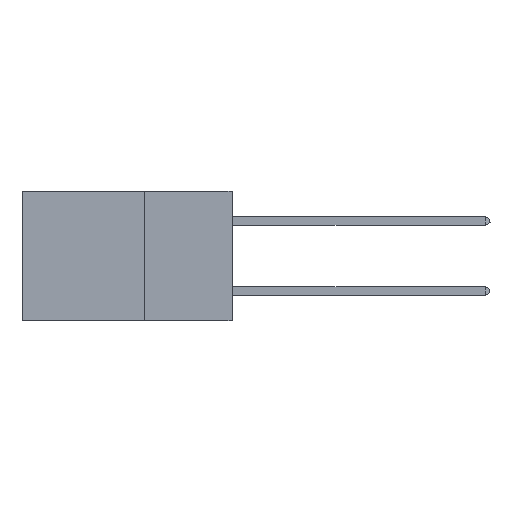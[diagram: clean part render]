
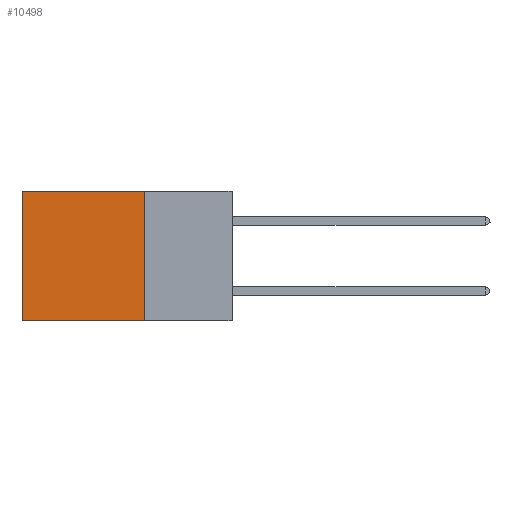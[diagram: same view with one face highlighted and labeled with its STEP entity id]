
A CAD part, left-side view. The second image highlights one B-rep face of the part: STEP entity #10498.
In plain terms, the highlighted planar face has unit normal (-1, 0, 0).
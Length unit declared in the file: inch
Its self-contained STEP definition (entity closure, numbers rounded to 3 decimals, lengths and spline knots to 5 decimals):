
#147 = VECTOR ( 'NONE', #10610, 39.37008 ) ;
#389 = CARTESIAN_POINT ( 'NONE',  ( 0.2875, 0.6, 0. ) ) ;
#582 = CARTESIAN_POINT ( 'NONE',  ( 0.2875, 0.6, 0. ) ) ;
#1694 = VERTEX_POINT ( 'NONE', #389 ) ;
#1962 = CARTESIAN_POINT ( 'NONE',  ( 0.2875, 0.25, 0. ) ) ;
#3839 = LINE ( 'NONE', #1962, #12607 ) ;
#4952 = CARTESIAN_POINT ( 'NONE',  ( 0.2875, 0.6, -0.37 ) ) ;
#6584 = LINE ( 'NONE', #582, #10654 ) ;
#7251 = AXIS2_PLACEMENT_3D ( 'NONE', #15501, #9727, #23366 ) ;
#8594 = CARTESIAN_POINT ( 'NONE',  ( 0.2875, 0.25, -0.37 ) ) ;
#9340 = DIRECTION ( 'NONE',  ( 0., 0., -1. ) ) ;
#9702 = LINE ( 'NONE', #19185, #13711 ) ;
#9727 = DIRECTION ( 'NONE',  ( 1., 0., 0. ) ) ;
#10261 = EDGE_CURVE ( 'NONE', #25436, #23892, #16090, .T. ) ;
#10397 = ORIENTED_EDGE ( 'NONE', *, *, #20619, .T. ) ;
#10498 = ADVANCED_FACE ( 'NONE', ( #15770 ), #21427, .F. ) ;
#10610 = DIRECTION ( 'NONE',  ( 0., 1., 0. ) ) ;
#10654 = VECTOR ( 'NONE', #22195, 39.37008 ) ;
#12137 = VERTEX_POINT ( 'NONE', #22194 ) ;
#12607 = VECTOR ( 'NONE', #13898, 39.37008 ) ;
#13711 = VECTOR ( 'NONE', #9340, 39.37008 ) ;
#13855 = ORIENTED_EDGE ( 'NONE', *, *, #22346, .T. ) ;
#13898 = DIRECTION ( 'NONE',  ( 0., 1., 0. ) ) ;
#15501 = CARTESIAN_POINT ( 'NONE',  ( 0.2875, 0.25, 0. ) ) ;
#15770 = FACE_OUTER_BOUND ( 'NONE', #16786, .T. ) ;
#16090 = LINE ( 'NONE', #8594, #147 ) ;
#16786 = EDGE_LOOP ( 'NONE', ( #10397, #24883, #20559, #13855 ) ) ;
#19185 = CARTESIAN_POINT ( 'NONE',  ( 0.2875, 0.25, 0. ) ) ;
#20559 = ORIENTED_EDGE ( 'NONE', *, *, #21579, .F. ) ;
#20619 = EDGE_CURVE ( 'NONE', #1694, #23892, #6584, .T. ) ;
#21427 = PLANE ( 'NONE',  #7251 ) ;
#21579 = EDGE_CURVE ( 'NONE', #12137, #25436, #9702, .T. ) ;
#22194 = CARTESIAN_POINT ( 'NONE',  ( 0.2875, 0.25, 0. ) ) ;
#22195 = DIRECTION ( 'NONE',  ( 0., 0., -1. ) ) ;
#22346 = EDGE_CURVE ( 'NONE', #12137, #1694, #3839, .T. ) ;
#23366 = DIRECTION ( 'NONE',  ( 0., 0., -1. ) ) ;
#23892 = VERTEX_POINT ( 'NONE', #4952 ) ;
#24883 = ORIENTED_EDGE ( 'NONE', *, *, #10261, .F. ) ;
#25079 = CARTESIAN_POINT ( 'NONE',  ( 0.2875, 0.25, -0.37 ) ) ;
#25436 = VERTEX_POINT ( 'NONE', #25079 ) ;
